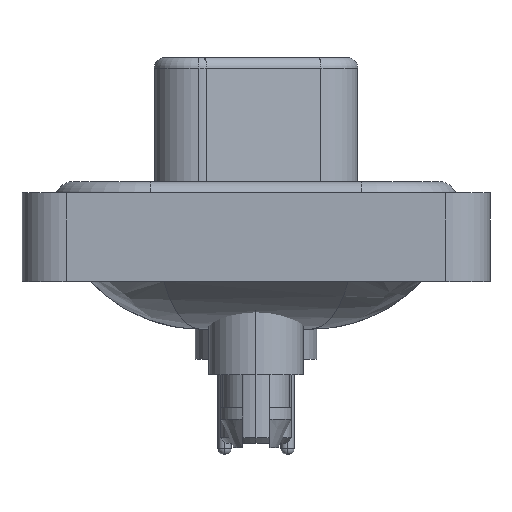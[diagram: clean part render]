
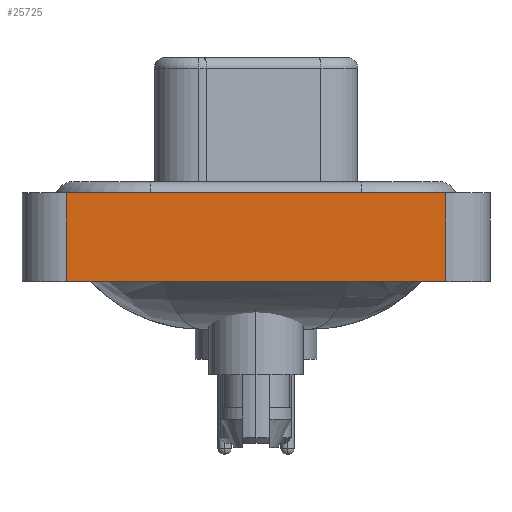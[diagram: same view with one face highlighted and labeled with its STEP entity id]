
A CAD part, left-side view. The second image highlights one B-rep face of the part: STEP entity #25725.
In plain terms, the highlighted planar face has unit normal (-1, 0, 0).
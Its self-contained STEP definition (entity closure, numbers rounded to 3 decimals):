
#1230 = VECTOR ( 'NONE', #20872, 1000. ) ;
#1887 = EDGE_LOOP ( 'NONE', ( #20220, #19425, #23946, #5255 ) ) ;
#2082 = LINE ( 'NONE', #20856, #9941 ) ;
#2340 = CARTESIAN_POINT ( 'NONE',  ( -7.35, -8.55, -3.6 ) ) ;
#2483 = VERTEX_POINT ( 'NONE', #9457 ) ;
#3750 = DIRECTION ( 'NONE',  ( -1., 0., 0. ) ) ;
#4286 = CARTESIAN_POINT ( 'NONE',  ( -7.35, -8.55, 0.4 ) ) ;
#4668 = DIRECTION ( 'NONE',  ( 0., -1., 0. ) ) ;
#5049 = VERTEX_POINT ( 'NONE', #6558 ) ;
#5255 = ORIENTED_EDGE ( 'NONE', *, *, #7924, .T. ) ;
#5659 = CARTESIAN_POINT ( 'NONE',  ( -7.35, -8.55, -3.6 ) ) ;
#6558 = CARTESIAN_POINT ( 'NONE',  ( -7.35, 8.55, 0.4 ) ) ;
#6685 = LINE ( 'NONE', #2340, #11162 ) ;
#7721 = DIRECTION ( 'NONE',  ( 0., 0., 1. ) ) ;
#7924 = EDGE_CURVE ( 'NONE', #23304, #10022, #6685, .T. ) ;
#9457 = CARTESIAN_POINT ( 'NONE',  ( -7.35, -8.55, 0.4 ) ) ;
#9765 = CARTESIAN_POINT ( 'NONE',  ( -7.35, 8.55, -3.6 ) ) ;
#9890 = PLANE ( 'NONE',  #10543 ) ;
#9941 = VECTOR ( 'NONE', #16757, 1000. ) ;
#10022 = VERTEX_POINT ( 'NONE', #23439 ) ;
#10143 = DIRECTION ( 'NONE',  ( 0., 0., 1. ) ) ;
#10310 = VECTOR ( 'NONE', #7721, 1000. ) ;
#10543 = AXIS2_PLACEMENT_3D ( 'NONE', #5659, #3750, #10143 ) ;
#11144 = EDGE_CURVE ( 'NONE', #5049, #2483, #24673, .T. ) ;
#11162 = VECTOR ( 'NONE', #4668, 1000. ) ;
#16757 = DIRECTION ( 'NONE',  ( 0., 0., 1. ) ) ;
#18302 = LINE ( 'NONE', #9765, #10310 ) ;
#19425 = ORIENTED_EDGE ( 'NONE', *, *, #11144, .F. ) ;
#20220 = ORIENTED_EDGE ( 'NONE', *, *, #24329, .T. ) ;
#20856 = CARTESIAN_POINT ( 'NONE',  ( -7.35, -8.55, -3.6 ) ) ;
#20872 = DIRECTION ( 'NONE',  ( 0., -1., 0. ) ) ;
#21793 = CARTESIAN_POINT ( 'NONE',  ( -7.35, 8.55, -3.6 ) ) ;
#22245 = FACE_OUTER_BOUND ( 'NONE', #1887, .T. ) ;
#22248 = EDGE_CURVE ( 'NONE', #23304, #5049, #18302, .T. ) ;
#23304 = VERTEX_POINT ( 'NONE', #21793 ) ;
#23439 = CARTESIAN_POINT ( 'NONE',  ( -7.35, -8.55, -3.6 ) ) ;
#23946 = ORIENTED_EDGE ( 'NONE', *, *, #22248, .F. ) ;
#24329 = EDGE_CURVE ( 'NONE', #10022, #2483, #2082, .T. ) ;
#24673 = LINE ( 'NONE', #4286, #1230 ) ;
#25725 = ADVANCED_FACE ( 'NONE', ( #22245 ), #9890, .T. ) ;
